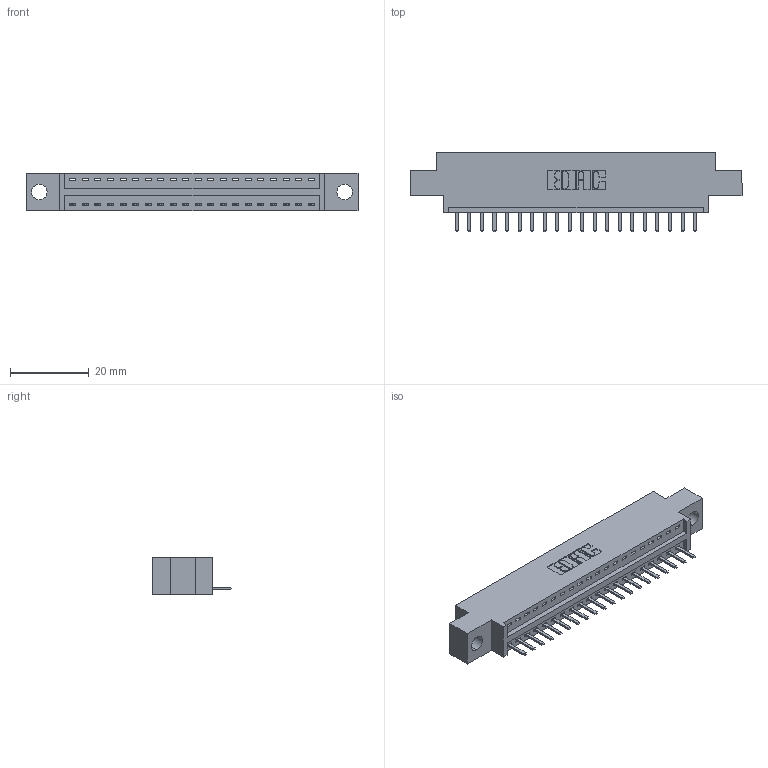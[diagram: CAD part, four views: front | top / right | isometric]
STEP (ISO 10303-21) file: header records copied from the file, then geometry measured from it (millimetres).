
FILE_DESCRIPTION (( 'STEP AP203' ), '1' );
FILE_NAME ('346-020-520-604.STEP', '2022-05-05T16:16:12', ( '' ), ( '' ), 'SwSTEP 2.0', 'SolidWorks 2020', '' );
FILE_SCHEMA (( 'CONFIG_CONTROL_DESIGN' ));
Length unit declared in the file: inch
Products named in the file (3): 346-020-520-604; 345-292-001_345-293-120; 346 Part_0.170 Offset - 0.156 Dia-TH
Assembly tree (21 placements, depth 2):
  346-020-520-604
    346 Part_0.170 Offset - 0.156 Dia-TH
    345-292-001_345-293-120  x20
Bounding box: 84.07 x 20.02 x 9.4 mm (x, y, z)
Volume: 7578.1 mm3; surface area: 9039.8 mm2
Topology: 21 solids, 21 shells, 1380 faces, 4057 edges, 2650 vertices
Faces by surface type: plane 934, cylinder 446
Entity records: 16039 total; most frequent: CARTESIAN_POINT 2778, ORIENTED_EDGE 2718, DIRECTION 2463, EDGE_CURVE 1359, LINE 1143, VECTOR 1143, VERTEX_POINT 902, AXIS2_PLACEMENT_3D 660
